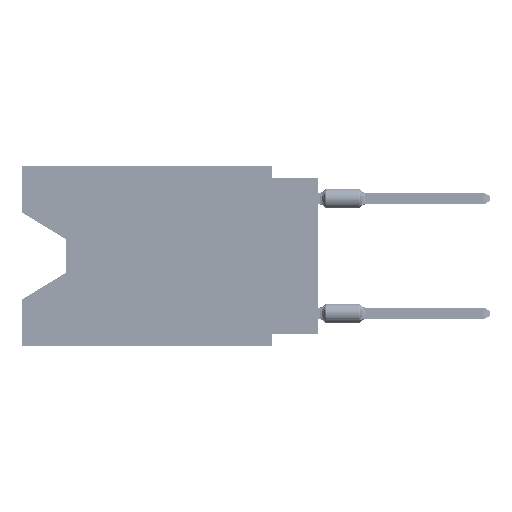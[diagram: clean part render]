
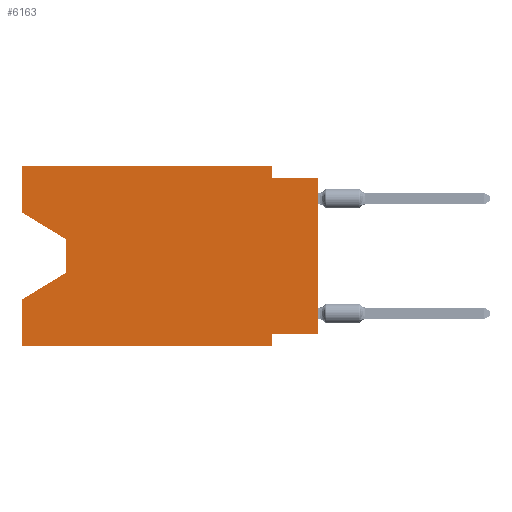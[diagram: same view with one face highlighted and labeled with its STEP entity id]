
A CAD part, left-side view. The second image highlights one B-rep face of the part: STEP entity #6163.
In plain terms, the highlighted planar face has unit normal (-1, 0, 0).
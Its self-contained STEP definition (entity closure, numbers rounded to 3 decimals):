
#154 = EDGE_CURVE ( 'NONE', #47693, #43353, #56988, .T. ) ;
#2984 = VECTOR ( 'NONE', #5203, 1000. ) ;
#3110 = ORIENTED_EDGE ( 'NONE', *, *, #19120, .T. ) ;
#3275 = DIRECTION ( 'NONE',  ( 0., 0., -1. ) ) ;
#3396 = CARTESIAN_POINT ( 'NONE',  ( 0., 16.383, -2.546 ) ) ;
#3476 = EDGE_CURVE ( 'NONE', #67492, #9462, #62165, .T. ) ;
#3529 = LINE ( 'NONE', #40878, #5342 ) ;
#4670 = LINE ( 'NONE', #58771, #66808 ) ;
#4782 = VERTEX_POINT ( 'NONE', #10566 ) ;
#4936 = CARTESIAN_POINT ( 'NONE',  ( 0., 16.383, 0. ) ) ;
#5203 = DIRECTION ( 'NONE',  ( 0., -1., 0. ) ) ;
#5342 = VECTOR ( 'NONE', #20299, 1000. ) ;
#6136 = CARTESIAN_POINT ( 'NONE',  ( 0., 16.383, 0. ) ) ;
#6163 = ADVANCED_FACE ( 'NONE', ( #6326 ), #42992, .F. ) ;
#6326 = FACE_OUTER_BOUND ( 'NONE', #17440, .T. ) ;
#6505 = VECTOR ( 'NONE', #21860, 1000. ) ;
#6755 = DIRECTION ( 'NONE',  ( 0., -1., 0. ) ) ;
#6797 = EDGE_CURVE ( 'NONE', #34835, #21042, #11839, .T. ) ;
#7300 = CARTESIAN_POINT ( 'NONE',  ( 0., 16.383, -9.906 ) ) ;
#8211 = CARTESIAN_POINT ( 'NONE',  ( 0., 0., -0.635 ) ) ;
#8491 = ORIENTED_EDGE ( 'NONE', *, *, #49930, .F. ) ;
#9462 = VERTEX_POINT ( 'NONE', #36233 ) ;
#10566 = CARTESIAN_POINT ( 'NONE',  ( 0., 2.54, 0. ) ) ;
#11839 = LINE ( 'NONE', #33129, #35793 ) ;
#12115 = EDGE_CURVE ( 'NONE', #23007, #4782, #47625, .T. ) ;
#14282 = ORIENTED_EDGE ( 'NONE', *, *, #26982, .F. ) ;
#14310 = VERTEX_POINT ( 'NONE', #21080 ) ;
#14358 = CARTESIAN_POINT ( 'NONE',  ( 0., 16.383, 0. ) ) ;
#16437 = VECTOR ( 'NONE', #26256, 1000. ) ;
#17440 = EDGE_LOOP ( 'NONE', ( #3110, #30008, #37618, #21176, #57951, #8491, #54035, #42345, #42698, #14282, #62597, #67434 ) ) ;
#17476 = EDGE_CURVE ( 'NONE', #67492, #19320, #20936, .T. ) ;
#18396 = CARTESIAN_POINT ( 'NONE',  ( 0., 2.54, -0.635 ) ) ;
#19120 = EDGE_CURVE ( 'NONE', #46111, #14310, #51222, .T. ) ;
#19142 = VECTOR ( 'NONE', #6755, 1000. ) ;
#19320 = VERTEX_POINT ( 'NONE', #38599 ) ;
#19694 = CARTESIAN_POINT ( 'NONE',  ( 0., 2.54, 0. ) ) ;
#20299 = DIRECTION ( 'NONE',  ( 0., 0., 1. ) ) ;
#20658 = DIRECTION ( 'NONE',  ( 0., 0.855, -0.519 ) ) ;
#20936 = LINE ( 'NONE', #32097, #2984 ) ;
#21042 = VERTEX_POINT ( 'NONE', #49348 ) ;
#21080 = CARTESIAN_POINT ( 'NONE',  ( 0., 13.97, -4.013 ) ) ;
#21176 = ORIENTED_EDGE ( 'NONE', *, *, #3476, .F. ) ;
#21860 = DIRECTION ( 'NONE',  ( 0., 0., 1. ) ) ;
#22398 = DIRECTION ( 'NONE',  ( 1., 0., 0. ) ) ;
#23007 = VERTEX_POINT ( 'NONE', #68739 ) ;
#23910 = VECTOR ( 'NONE', #3275, 1000. ) ;
#25976 = DIRECTION ( 'NONE',  ( 0., 0., -1. ) ) ;
#26256 = DIRECTION ( 'NONE',  ( 0., -1., 0. ) ) ;
#26405 = LINE ( 'NONE', #6136, #6505 ) ;
#26982 = EDGE_CURVE ( 'NONE', #4782, #47693, #67518, .T. ) ;
#29193 = CARTESIAN_POINT ( 'NONE',  ( 0., 13.97, -5.893 ) ) ;
#30008 = ORIENTED_EDGE ( 'NONE', *, *, #36337, .T. ) ;
#31833 = VECTOR ( 'NONE', #20658, 1000. ) ;
#31883 = EDGE_CURVE ( 'NONE', #46111, #23007, #26405, .T. ) ;
#32097 = CARTESIAN_POINT ( 'NONE',  ( 0., 16.383, -9.906 ) ) ;
#33129 = CARTESIAN_POINT ( 'NONE',  ( 0., 0., -9.271 ) ) ;
#33949 = DIRECTION ( 'NONE',  ( 0., 0., -1. ) ) ;
#34514 = DIRECTION ( 'NONE',  ( 0., 1., 0. ) ) ;
#34835 = VERTEX_POINT ( 'NONE', #46207 ) ;
#35793 = VECTOR ( 'NONE', #34514, 1000. ) ;
#36233 = CARTESIAN_POINT ( 'NONE',  ( 0., 16.383, -7.36 ) ) ;
#36337 = EDGE_CURVE ( 'NONE', #14310, #44387, #45806, .T. ) ;
#37618 = ORIENTED_EDGE ( 'NONE', *, *, #41960, .T. ) ;
#38439 = DIRECTION ( 'NONE',  ( 0., 0., -1. ) ) ;
#38599 = CARTESIAN_POINT ( 'NONE',  ( 0., 2.54, -9.906 ) ) ;
#40878 = CARTESIAN_POINT ( 'NONE',  ( 0., 0., 0. ) ) ;
#41101 = DIRECTION ( 'NONE',  ( 0., -0.855, -0.519 ) ) ;
#41549 = DIRECTION ( 'NONE',  ( 0., 0., 1. ) ) ;
#41960 = EDGE_CURVE ( 'NONE', #44387, #9462, #67814, .T. ) ;
#42345 = ORIENTED_EDGE ( 'NONE', *, *, #48613, .T. ) ;
#42417 = AXIS2_PLACEMENT_3D ( 'NONE', #4936, #22398, #38439 ) ;
#42698 = ORIENTED_EDGE ( 'NONE', *, *, #154, .F. ) ;
#42992 = PLANE ( 'NONE',  #42417 ) ;
#43353 = VERTEX_POINT ( 'NONE', #8211 ) ;
#44387 = VERTEX_POINT ( 'NONE', #29193 ) ;
#45368 = VECTOR ( 'NONE', #41101, 1000. ) ;
#45806 = LINE ( 'NONE', #61190, #62987 ) ;
#46111 = VERTEX_POINT ( 'NONE', #46704 ) ;
#46207 = CARTESIAN_POINT ( 'NONE',  ( 0., 0., -9.271 ) ) ;
#46704 = CARTESIAN_POINT ( 'NONE',  ( 0., 16.383, -2.546 ) ) ;
#47625 = LINE ( 'NONE', #68938, #19142 ) ;
#47693 = VERTEX_POINT ( 'NONE', #18396 ) ;
#48613 = EDGE_CURVE ( 'NONE', #34835, #43353, #3529, .T. ) ;
#49348 = CARTESIAN_POINT ( 'NONE',  ( 0., 2.54, -9.271 ) ) ;
#49930 = EDGE_CURVE ( 'NONE', #21042, #19320, #4670, .T. ) ;
#51222 = LINE ( 'NONE', #3396, #45368 ) ;
#51747 = CARTESIAN_POINT ( 'NONE',  ( 0., 0., -0.635 ) ) ;
#52383 = VECTOR ( 'NONE', #41549, 1000. ) ;
#54035 = ORIENTED_EDGE ( 'NONE', *, *, #6797, .F. ) ;
#56988 = LINE ( 'NONE', #51747, #16437 ) ;
#57951 = ORIENTED_EDGE ( 'NONE', *, *, #17476, .T. ) ;
#58771 = CARTESIAN_POINT ( 'NONE',  ( 0., 2.54, -9.906 ) ) ;
#61190 = CARTESIAN_POINT ( 'NONE',  ( 0., 13.97, -4.013 ) ) ;
#62165 = LINE ( 'NONE', #14358, #52383 ) ;
#62227 = CARTESIAN_POINT ( 'NONE',  ( 0., 13.97, -5.893 ) ) ;
#62597 = ORIENTED_EDGE ( 'NONE', *, *, #12115, .F. ) ;
#62987 = VECTOR ( 'NONE', #33949, 1000. ) ;
#66808 = VECTOR ( 'NONE', #25976, 1000. ) ;
#67434 = ORIENTED_EDGE ( 'NONE', *, *, #31883, .F. ) ;
#67492 = VERTEX_POINT ( 'NONE', #7300 ) ;
#67518 = LINE ( 'NONE', #19694, #23910 ) ;
#67814 = LINE ( 'NONE', #62227, #31833 ) ;
#68739 = CARTESIAN_POINT ( 'NONE',  ( 0., 16.383, 0. ) ) ;
#68938 = CARTESIAN_POINT ( 'NONE',  ( 0., 16.383, 0. ) ) ;
